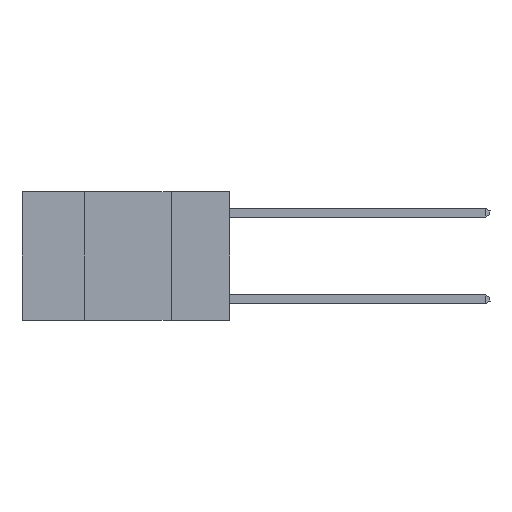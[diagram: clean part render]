
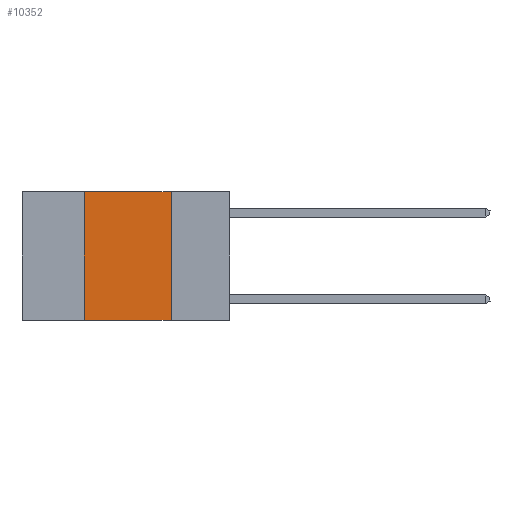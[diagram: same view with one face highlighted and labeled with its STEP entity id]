
A CAD part, left-side view. The second image highlights one B-rep face of the part: STEP entity #10352.
In plain terms, the highlighted planar face has unit normal (-1, 0, 0).
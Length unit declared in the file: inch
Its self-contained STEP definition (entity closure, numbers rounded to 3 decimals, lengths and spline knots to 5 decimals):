
#60 = VERTEX_POINT ( 'NONE', #9484 ) ;
#381 = DIRECTION ( 'NONE',  ( 0., 0., 1. ) ) ;
#662 = VERTEX_POINT ( 'NONE', #6310 ) ;
#1048 = FACE_OUTER_BOUND ( 'NONE', #3910, .T. ) ;
#1348 = EDGE_CURVE ( 'NONE', #11898, #662, #2888, .T. ) ;
#1715 = DIRECTION ( 'NONE',  ( 0., -1., 0. ) ) ;
#1719 = CARTESIAN_POINT ( 'NONE',  ( 0., 0.6, 0. ) ) ;
#2021 = CARTESIAN_POINT ( 'NONE',  ( 0., 0.17, 0. ) ) ;
#2691 = CARTESIAN_POINT ( 'NONE',  ( 0., 0.6, 0. ) ) ;
#2888 = LINE ( 'NONE', #1719, #12176 ) ;
#2974 = VECTOR ( 'NONE', #1715, 39.37008 ) ;
#3761 = LINE ( 'NONE', #2021, #8902 ) ;
#3910 = EDGE_LOOP ( 'NONE', ( #9369, #10330, #9542, #3918 ) ) ;
#3918 = ORIENTED_EDGE ( 'NONE', *, *, #9695, .T. ) ;
#4333 = EDGE_CURVE ( 'NONE', #662, #5859, #3761, .T. ) ;
#4739 = DIRECTION ( 'NONE',  ( 0., 0., -1. ) ) ;
#5859 = VERTEX_POINT ( 'NONE', #9930 ) ;
#6310 = CARTESIAN_POINT ( 'NONE',  ( 0., 0.17, 0. ) ) ;
#6730 = PLANE ( 'NONE',  #7323 ) ;
#6837 = VECTOR ( 'NONE', #381, 39.37008 ) ;
#7165 = LINE ( 'NONE', #10618, #6837 ) ;
#7323 = AXIS2_PLACEMENT_3D ( 'NONE', #2691, #10894, #4739 ) ;
#8429 = LINE ( 'NONE', #10909, #2974 ) ;
#8902 = VECTOR ( 'NONE', #11313, 39.37008 ) ;
#9369 = ORIENTED_EDGE ( 'NONE', *, *, #4333, .F. ) ;
#9484 = CARTESIAN_POINT ( 'NONE',  ( 0., 0.42, -0.37 ) ) ;
#9542 = ORIENTED_EDGE ( 'NONE', *, *, #12495, .F. ) ;
#9608 = CARTESIAN_POINT ( 'NONE',  ( 0., 0.42, 0. ) ) ;
#9695 = EDGE_CURVE ( 'NONE', #60, #5859, #8429, .T. ) ;
#9930 = CARTESIAN_POINT ( 'NONE',  ( 0., 0.17, -0.37 ) ) ;
#10330 = ORIENTED_EDGE ( 'NONE', *, *, #1348, .F. ) ;
#10352 = ADVANCED_FACE ( 'NONE', ( #1048 ), #6730, .F. ) ;
#10618 = CARTESIAN_POINT ( 'NONE',  ( 0., 0.42, 0. ) ) ;
#10750 = DIRECTION ( 'NONE',  ( 0., -1., 0. ) ) ;
#10894 = DIRECTION ( 'NONE',  ( 1., 0., 0. ) ) ;
#10909 = CARTESIAN_POINT ( 'NONE',  ( 0., 0.6, -0.37 ) ) ;
#11313 = DIRECTION ( 'NONE',  ( 0., 0., -1. ) ) ;
#11898 = VERTEX_POINT ( 'NONE', #9608 ) ;
#12176 = VECTOR ( 'NONE', #10750, 39.37008 ) ;
#12495 = EDGE_CURVE ( 'NONE', #60, #11898, #7165, .T. ) ;
